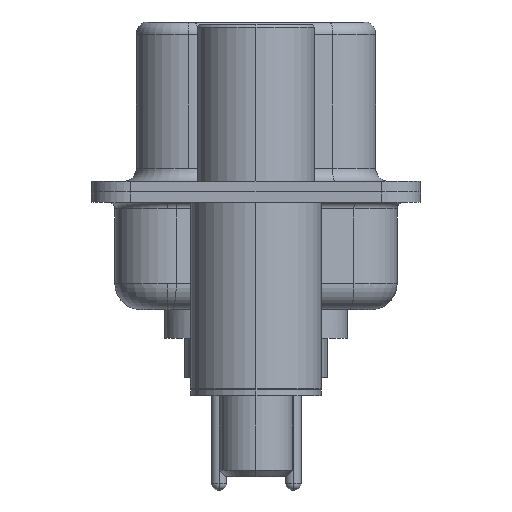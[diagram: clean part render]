
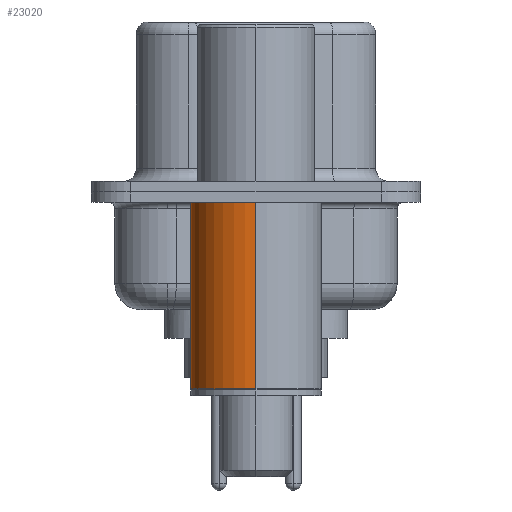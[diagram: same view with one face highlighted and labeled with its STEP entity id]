
A CAD part, left-side view. The second image highlights one B-rep face of the part: STEP entity #23020.
In plain terms, the highlighted cylindrical face has radius 2.5 mm (diameter 5 mm), a partial arc.
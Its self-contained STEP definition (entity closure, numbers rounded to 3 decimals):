
#558 = CARTESIAN_POINT ( 'NONE',  ( -2.5, 0., -7.525 ) ) ;
#1249 = VERTEX_POINT ( 'NONE', #19213 ) ;
#1350 = CYLINDRICAL_SURFACE ( 'NONE', #17559, 2.5 ) ;
#1863 = DIRECTION ( 'NONE',  ( 0., 0., 1. ) ) ;
#2530 = DIRECTION ( 'NONE',  ( 0., 0., 1. ) ) ;
#2777 = CIRCLE ( 'NONE', #17744, 2.5 ) ;
#5741 = DIRECTION ( 'NONE',  ( 1., 0., 0. ) ) ;
#5937 = VECTOR ( 'NONE', #19004, 1000. ) ;
#6813 = ORIENTED_EDGE ( 'NONE', *, *, #16119, .F. ) ;
#6853 = FACE_OUTER_BOUND ( 'NONE', #20370, .T. ) ;
#8243 = ORIENTED_EDGE ( 'NONE', *, *, #15892, .T. ) ;
#9164 = VERTEX_POINT ( 'NONE', #22376 ) ;
#10438 = CARTESIAN_POINT ( 'NONE',  ( 2.5, 0., -0.4 ) ) ;
#10837 = ORIENTED_EDGE ( 'NONE', *, *, #15624, .F. ) ;
#13082 = CARTESIAN_POINT ( 'NONE',  ( 0., 0., -7.525 ) ) ;
#13760 = CARTESIAN_POINT ( 'NONE',  ( 0., 0., -0.4 ) ) ;
#14278 = DIRECTION ( 'NONE',  ( 0., 0., 1. ) ) ;
#15011 = DIRECTION ( 'NONE',  ( 1., 0., 0. ) ) ;
#15624 = EDGE_CURVE ( 'NONE', #1249, #17303, #18666, .T. ) ;
#15656 = DIRECTION ( 'NONE',  ( 1., 0., 0. ) ) ;
#15892 = EDGE_CURVE ( 'NONE', #1249, #22357, #2777, .T. ) ;
#15969 = LINE ( 'NONE', #20853, #5937 ) ;
#15973 = EDGE_CURVE ( 'NONE', #22357, #9164, #15969, .T. ) ;
#15981 = ORIENTED_EDGE ( 'NONE', *, *, #15973, .T. ) ;
#16119 = EDGE_CURVE ( 'NONE', #17303, #9164, #24115, .T. ) ;
#16873 = VECTOR ( 'NONE', #14278, 1000. ) ;
#17049 = DIRECTION ( 'NONE',  ( 0., 0., 1. ) ) ;
#17269 = AXIS2_PLACEMENT_3D ( 'NONE', #13760, #2530, #15656 ) ;
#17303 = VERTEX_POINT ( 'NONE', #10438 ) ;
#17559 = AXIS2_PLACEMENT_3D ( 'NONE', #22612, #17049, #5741 ) ;
#17744 = AXIS2_PLACEMENT_3D ( 'NONE', #13082, #1863, #15011 ) ;
#18666 = LINE ( 'NONE', #19987, #16873 ) ;
#19004 = DIRECTION ( 'NONE',  ( 0., 0., 1. ) ) ;
#19213 = CARTESIAN_POINT ( 'NONE',  ( 2.5, 0., -7.525 ) ) ;
#19987 = CARTESIAN_POINT ( 'NONE',  ( 2.5, 0., 0.581 ) ) ;
#20370 = EDGE_LOOP ( 'NONE', ( #8243, #15981, #6813, #10837 ) ) ;
#20853 = CARTESIAN_POINT ( 'NONE',  ( -2.5, 0., 0.581 ) ) ;
#22357 = VERTEX_POINT ( 'NONE', #558 ) ;
#22376 = CARTESIAN_POINT ( 'NONE',  ( -2.5, 0., -0.4 ) ) ;
#22612 = CARTESIAN_POINT ( 'NONE',  ( 0., 0., 0.581 ) ) ;
#23020 = ADVANCED_FACE ( 'NONE', ( #6853 ), #1350, .T. ) ;
#24115 = CIRCLE ( 'NONE', #17269, 2.5 ) ;
